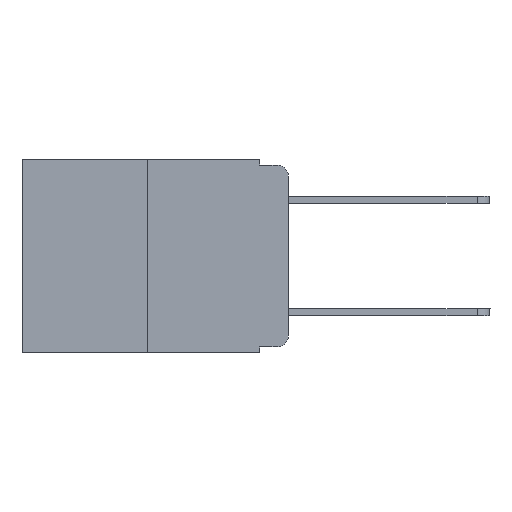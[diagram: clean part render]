
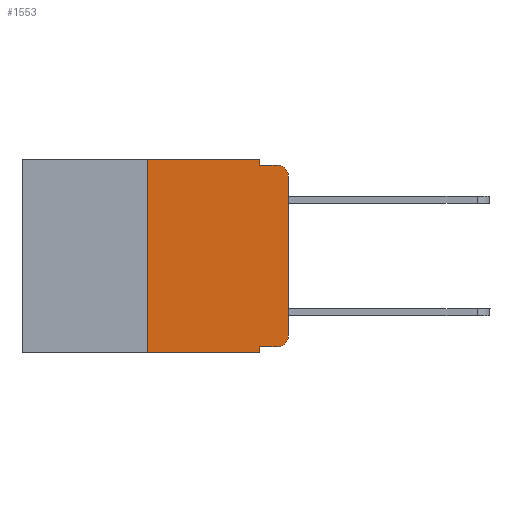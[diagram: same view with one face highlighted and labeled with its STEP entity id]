
A CAD part, left-side view. The second image highlights one B-rep face of the part: STEP entity #1553.
In plain terms, the highlighted planar face has unit normal (-1, 0, 0).
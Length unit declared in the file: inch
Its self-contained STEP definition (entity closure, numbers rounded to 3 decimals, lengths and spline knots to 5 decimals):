
#95 = ORIENTED_EDGE ( 'NONE', *, *, #4016, .F. ) ;
#118 = VERTEX_POINT ( 'NONE', #5402 ) ;
#347 = ORIENTED_EDGE ( 'NONE', *, *, #6268, .F. ) ;
#366 = DIRECTION ( 'NONE',  ( 0., 0., -1. ) ) ;
#507 = CARTESIAN_POINT ( 'NONE',  ( 0., 0., 0. ) ) ;
#685 = CARTESIAN_POINT ( 'NONE',  ( 0., 0.051, 0. ) ) ;
#937 = ORIENTED_EDGE ( 'NONE', *, *, #5140, .T. ) ;
#1001 = CARTESIAN_POINT ( 'NONE',  ( 0., 0.051, -0.333 ) ) ;
#1553 = ADVANCED_FACE ( 'NONE', ( #11126 ), #5735, .F. ) ;
#1657 = DIRECTION ( 'NONE',  ( 0., 0., -1. ) ) ;
#1832 = CARTESIAN_POINT ( 'NONE',  ( 0., 0.051, -0.343 ) ) ;
#1921 = LINE ( 'NONE', #6741, #3040 ) ;
#1959 = AXIS2_PLACEMENT_3D ( 'NONE', #10011, #11652, #5434 ) ;
#2019 = EDGE_CURVE ( 'NONE', #5574, #11250, #5877, .T. ) ;
#2193 = CARTESIAN_POINT ( 'NONE',  ( 0., 0.051, -0.333 ) ) ;
#2396 = CARTESIAN_POINT ( 'NONE',  ( 0., 0.051, -0.01 ) ) ;
#2414 = ORIENTED_EDGE ( 'NONE', *, *, #3226, .F. ) ;
#2467 = LINE ( 'NONE', #8822, #3451 ) ;
#2686 = DIRECTION ( 'NONE',  ( 0., -1., 0. ) ) ;
#2708 = LINE ( 'NONE', #10001, #8805 ) ;
#2719 = LINE ( 'NONE', #507, #7683 ) ;
#2860 = LINE ( 'NONE', #5936, #8967 ) ;
#2991 = ORIENTED_EDGE ( 'NONE', *, *, #5503, .F. ) ;
#3008 = DIRECTION ( 'NONE',  ( 0., 0., -1. ) ) ;
#3040 = VECTOR ( 'NONE', #7668, 39.37008 ) ;
#3226 = EDGE_CURVE ( 'NONE', #118, #3594, #2708, .T. ) ;
#3418 = CARTESIAN_POINT ( 'NONE',  ( 0., 0.02, -0.313 ) ) ;
#3451 = VECTOR ( 'NONE', #5247, 39.37008 ) ;
#3594 = VERTEX_POINT ( 'NONE', #7018 ) ;
#3630 = EDGE_CURVE ( 'NONE', #7764, #8778, #6963, .T. ) ;
#3943 = CARTESIAN_POINT ( 'NONE',  ( 0., 0.473, 0. ) ) ;
#4003 = CARTESIAN_POINT ( 'NONE',  ( 0., 0., -0.03 ) ) ;
#4016 = EDGE_CURVE ( 'NONE', #8192, #11385, #1921, .T. ) ;
#4149 = EDGE_LOOP ( 'NONE', ( #10378, #8446, #347, #95, #2991, #2414, #7419, #7069, #937, #6373 ) ) ;
#4253 = AXIS2_PLACEMENT_3D ( 'NONE', #3943, #10286, #366 ) ;
#4707 = VECTOR ( 'NONE', #3008, 39.37008 ) ;
#5129 = EDGE_CURVE ( 'NONE', #9623, #5235, #8136, .T. ) ;
#5140 = EDGE_CURVE ( 'NONE', #5574, #7764, #10965, .T. ) ;
#5235 = VERTEX_POINT ( 'NONE', #6223 ) ;
#5247 = DIRECTION ( 'NONE',  ( 0., -1., 0. ) ) ;
#5402 = CARTESIAN_POINT ( 'NONE',  ( 0., 0.25, -0.343 ) ) ;
#5434 = DIRECTION ( 'NONE',  ( 0., 0., -1. ) ) ;
#5503 = EDGE_CURVE ( 'NONE', #3594, #8192, #2860, .T. ) ;
#5574 = VERTEX_POINT ( 'NONE', #2193 ) ;
#5724 = CARTESIAN_POINT ( 'NONE',  ( 0., 0.051, 0. ) ) ;
#5735 = PLANE ( 'NONE',  #4253 ) ;
#5877 = LINE ( 'NONE', #5724, #4707 ) ;
#5936 = CARTESIAN_POINT ( 'NONE',  ( 0., 0.473, 0. ) ) ;
#6223 = CARTESIAN_POINT ( 'NONE',  ( 0., 0.02, -0.01 ) ) ;
#6268 = EDGE_CURVE ( 'NONE', #11385, #5235, #11358, .T. ) ;
#6373 = ORIENTED_EDGE ( 'NONE', *, *, #3630, .T. ) ;
#6597 = EDGE_CURVE ( 'NONE', #8778, #9623, #2719, .T. ) ;
#6741 = CARTESIAN_POINT ( 'NONE',  ( 0., 0.051, 0. ) ) ;
#6938 = DIRECTION ( 'NONE',  ( 0., 0., 1. ) ) ;
#6963 = CIRCLE ( 'NONE', #10436, 0.02 ) ;
#7018 = CARTESIAN_POINT ( 'NONE',  ( 0., 0.25, 0. ) ) ;
#7069 = ORIENTED_EDGE ( 'NONE', *, *, #2019, .F. ) ;
#7419 = ORIENTED_EDGE ( 'NONE', *, *, #10521, .T. ) ;
#7668 = DIRECTION ( 'NONE',  ( 0., 0., -1. ) ) ;
#7683 = VECTOR ( 'NONE', #6938, 39.37008 ) ;
#7764 = VERTEX_POINT ( 'NONE', #8307 ) ;
#8136 = CIRCLE ( 'NONE', #1959, 0.02 ) ;
#8192 = VERTEX_POINT ( 'NONE', #685 ) ;
#8283 = VECTOR ( 'NONE', #2686, 39.37008 ) ;
#8307 = CARTESIAN_POINT ( 'NONE',  ( 0., 0.02, -0.333 ) ) ;
#8446 = ORIENTED_EDGE ( 'NONE', *, *, #5129, .T. ) ;
#8778 = VERTEX_POINT ( 'NONE', #9272 ) ;
#8805 = VECTOR ( 'NONE', #10922, 39.37008 ) ;
#8822 = CARTESIAN_POINT ( 'NONE',  ( 0., 0.473, -0.343 ) ) ;
#8967 = VECTOR ( 'NONE', #10379, 39.37008 ) ;
#9272 = CARTESIAN_POINT ( 'NONE',  ( 0., 0., -0.313 ) ) ;
#9623 = VERTEX_POINT ( 'NONE', #4003 ) ;
#9811 = VECTOR ( 'NONE', #11422, 39.37008 ) ;
#10001 = CARTESIAN_POINT ( 'NONE',  ( 0., 0.25, 0. ) ) ;
#10011 = CARTESIAN_POINT ( 'NONE',  ( 0., 0.02, -0.03 ) ) ;
#10286 = DIRECTION ( 'NONE',  ( 1., 0., 0. ) ) ;
#10378 = ORIENTED_EDGE ( 'NONE', *, *, #6597, .T. ) ;
#10379 = DIRECTION ( 'NONE',  ( 0., -1., 0. ) ) ;
#10436 = AXIS2_PLACEMENT_3D ( 'NONE', #3418, #11574, #1657 ) ;
#10521 = EDGE_CURVE ( 'NONE', #118, #11250, #2467, .T. ) ;
#10922 = DIRECTION ( 'NONE',  ( 0., 0., 1. ) ) ;
#10965 = LINE ( 'NONE', #1001, #8283 ) ;
#11126 = FACE_OUTER_BOUND ( 'NONE', #4149, .T. ) ;
#11250 = VERTEX_POINT ( 'NONE', #1832 ) ;
#11358 = LINE ( 'NONE', #2396, #9811 ) ;
#11385 = VERTEX_POINT ( 'NONE', #11662 ) ;
#11422 = DIRECTION ( 'NONE',  ( 0., -1., 0. ) ) ;
#11574 = DIRECTION ( 'NONE',  ( -1., 0., 0. ) ) ;
#11652 = DIRECTION ( 'NONE',  ( -1., 0., 0. ) ) ;
#11662 = CARTESIAN_POINT ( 'NONE',  ( 0., 0.051, -0.01 ) ) ;
